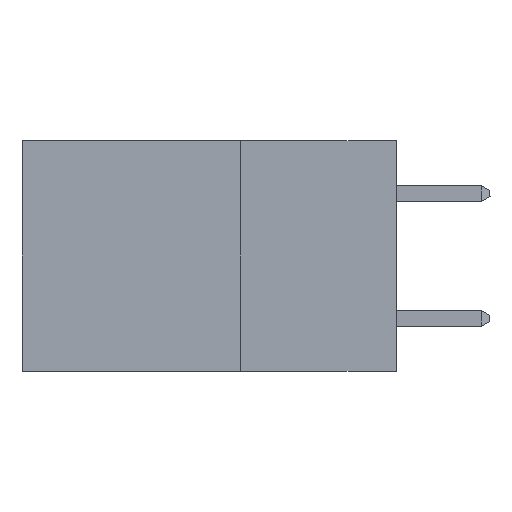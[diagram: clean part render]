
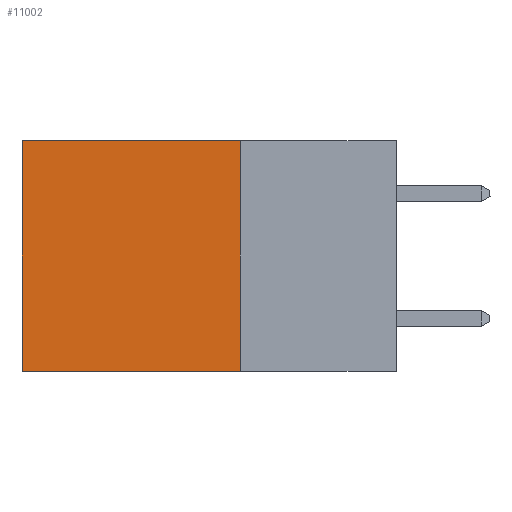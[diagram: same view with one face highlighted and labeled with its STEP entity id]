
A CAD part, left-side view. The second image highlights one B-rep face of the part: STEP entity #11002.
In plain terms, the highlighted planar face has unit normal (-1, 0, 0).
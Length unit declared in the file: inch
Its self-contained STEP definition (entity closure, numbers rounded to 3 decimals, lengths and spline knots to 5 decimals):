
#143 = LINE ( 'NONE', #19464, #1583 ) ;
#1330 = ORIENTED_EDGE ( 'NONE', *, *, #12109, .T. ) ;
#1525 = VERTEX_POINT ( 'NONE', #26445 ) ;
#1583 = VECTOR ( 'NONE', #12663, 39.37008 ) ;
#5221 = VECTOR ( 'NONE', #13083, 39.37008 ) ;
#5831 = EDGE_CURVE ( 'NONE', #14935, #1525, #9748, .T. ) ;
#6928 = VERTEX_POINT ( 'NONE', #26845 ) ;
#8555 = CARTESIAN_POINT ( 'NONE',  ( 0.298, 0.25, 0. ) ) ;
#9748 = LINE ( 'NONE', #27822, #21056 ) ;
#10287 = ORIENTED_EDGE ( 'NONE', *, *, #5831, .F. ) ;
#11002 = ADVANCED_FACE ( 'NONE', ( #17643 ), #23057, .F. ) ;
#11765 = CARTESIAN_POINT ( 'NONE',  ( 0.298, 0.25, 0. ) ) ;
#12109 = EDGE_CURVE ( 'NONE', #6928, #17779, #23271, .T. ) ;
#12663 = DIRECTION ( 'NONE',  ( 0., 0., -1. ) ) ;
#12727 = EDGE_CURVE ( 'NONE', #6928, #14935, #143, .T. ) ;
#12938 = AXIS2_PLACEMENT_3D ( 'NONE', #11765, #27594, #14032 ) ;
#13053 = DIRECTION ( 'NONE',  ( 0., 1., 0. ) ) ;
#13083 = DIRECTION ( 'NONE',  ( 0., 1., 0. ) ) ;
#14032 = DIRECTION ( 'NONE',  ( 0., 0., -1. ) ) ;
#14135 = EDGE_CURVE ( 'NONE', #17779, #1525, #21743, .T. ) ;
#14935 = VERTEX_POINT ( 'NONE', #18170 ) ;
#15447 = DIRECTION ( 'NONE',  ( 0., 0., -1. ) ) ;
#15716 = VECTOR ( 'NONE', #15447, 39.37008 ) ;
#16334 = ORIENTED_EDGE ( 'NONE', *, *, #12727, .F. ) ;
#17643 = FACE_OUTER_BOUND ( 'NONE', #19196, .T. ) ;
#17779 = VERTEX_POINT ( 'NONE', #20430 ) ;
#18170 = CARTESIAN_POINT ( 'NONE',  ( 0.298, 0.25, -0.37 ) ) ;
#19196 = EDGE_LOOP ( 'NONE', ( #27342, #10287, #16334, #1330 ) ) ;
#19464 = CARTESIAN_POINT ( 'NONE',  ( 0.298, 0.25, 0. ) ) ;
#20430 = CARTESIAN_POINT ( 'NONE',  ( 0.298, 0.6, 0. ) ) ;
#21056 = VECTOR ( 'NONE', #13053, 39.37008 ) ;
#21743 = LINE ( 'NONE', #29038, #15716 ) ;
#23057 = PLANE ( 'NONE',  #12938 ) ;
#23271 = LINE ( 'NONE', #8555, #5221 ) ;
#26445 = CARTESIAN_POINT ( 'NONE',  ( 0.298, 0.6, -0.37 ) ) ;
#26845 = CARTESIAN_POINT ( 'NONE',  ( 0.298, 0.25, 0. ) ) ;
#27342 = ORIENTED_EDGE ( 'NONE', *, *, #14135, .T. ) ;
#27594 = DIRECTION ( 'NONE',  ( 1., 0., 0. ) ) ;
#27822 = CARTESIAN_POINT ( 'NONE',  ( 0.298, 0.25, -0.37 ) ) ;
#29038 = CARTESIAN_POINT ( 'NONE',  ( 0.298, 0.6, 0. ) ) ;
